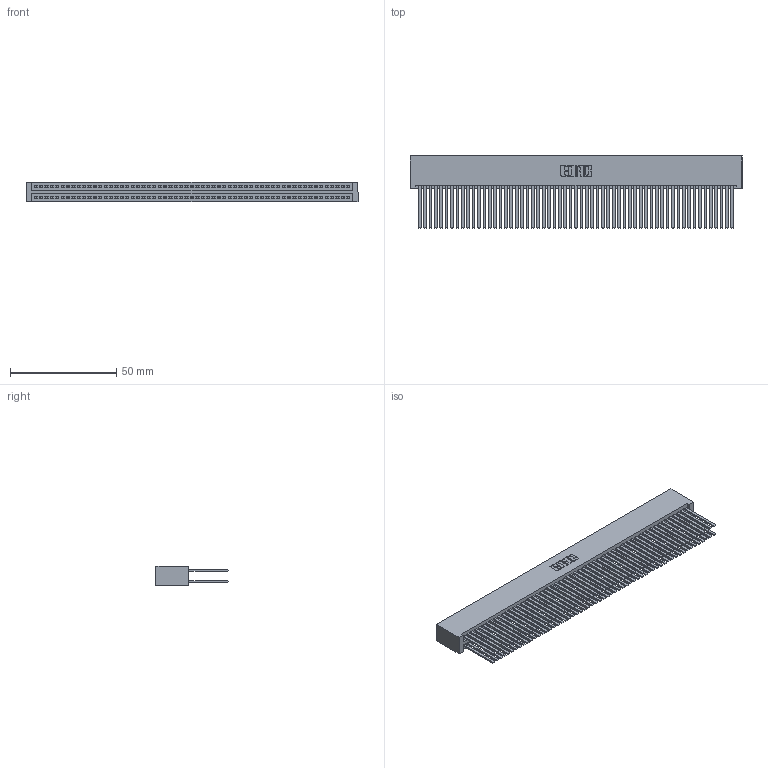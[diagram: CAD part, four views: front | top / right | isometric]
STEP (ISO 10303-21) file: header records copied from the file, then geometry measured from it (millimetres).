
FILE_DESCRIPTION (( 'STEP AP203' ), '1' );
FILE_NAME ('345-118-544-201.STEP', '2018-10-18T22:47:59', ( '' ), ( '' ), 'SwSTEP 2.0', 'SolidWorks 2016', '' );
FILE_SCHEMA (( 'CONFIG_CONTROL_DESIGN' ));
Length unit declared in the file: inch
Products named in the file (3): 345-118-544-201; 345-292-001_345-293-144; 345 Part_No Mounting Lugs
Assembly tree (119 placements, depth 2):
  345-118-544-201
    345 Part_No Mounting Lugs
    345-292-001_345-293-144  x118
Bounding box: 156.46 x 33.96 x 9.4 mm (x, y, z)
Volume: 17626.9 mm3; surface area: 31536.2 mm2
Topology: 119 solids, 119 shells, 5310 faces, 15775 edges, 10358 vertices
Faces by surface type: plane 3498, cylinder 1812
Entity records: 43543 total; most frequent: CARTESIAN_POINT 7280, ORIENTED_EDGE 7214, DIRECTION 6391, EDGE_CURVE 3607, VECTOR 3251, LINE 3251, VERTEX_POINT 2402, AXIS2_PLACEMENT_3D 1570
